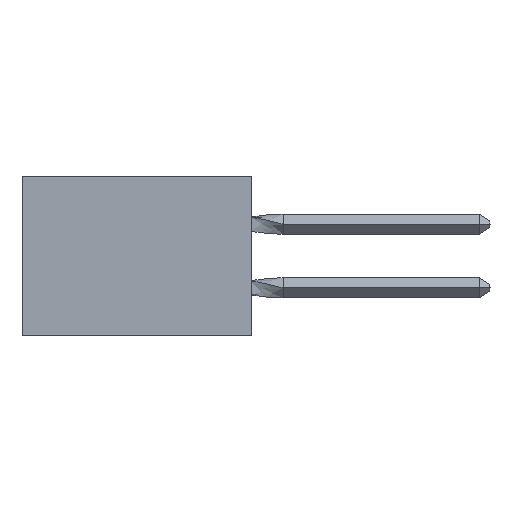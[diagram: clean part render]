
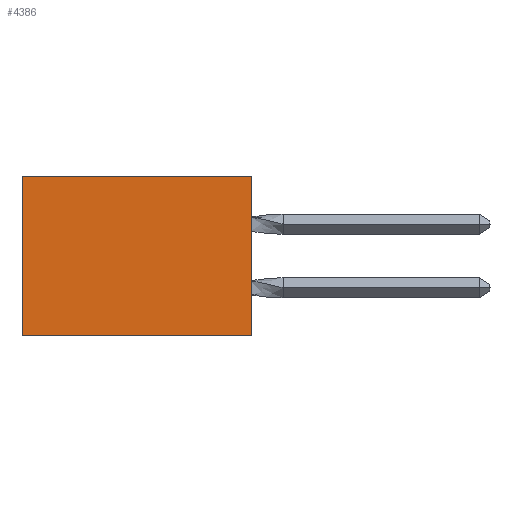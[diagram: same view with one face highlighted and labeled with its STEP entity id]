
A CAD part, left-side view. The second image highlights one B-rep face of the part: STEP entity #4386.
In plain terms, the highlighted planar face has unit normal (-1, 0, 0).
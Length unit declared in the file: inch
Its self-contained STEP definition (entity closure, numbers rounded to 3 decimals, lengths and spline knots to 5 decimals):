
#425 = ORIENTED_EDGE ( 'NONE', *, *, #20568, .T. ) ;
#957 = VERTEX_POINT ( 'NONE', #29753 ) ;
#1136 = LINE ( 'NONE', #21128, #17414 ) ;
#1670 = EDGE_CURVE ( 'NONE', #957, #11367, #22996, .T. ) ;
#1974 = DIRECTION ( 'NONE',  ( 1., 0., 0. ) ) ;
#3544 = DIRECTION ( 'NONE',  ( 0., 0., -1. ) ) ;
#3675 = ORIENTED_EDGE ( 'NONE', *, *, #31284, .F. ) ;
#4386 = ADVANCED_FACE ( 'NONE', ( #19103 ), #10804, .F. ) ;
#4981 = VERTEX_POINT ( 'NONE', #10867 ) ;
#6516 = VECTOR ( 'NONE', #23157, 39.37008 ) ;
#7247 = CARTESIAN_POINT ( 'NONE',  ( 0.305, 0., 0. ) ) ;
#10804 = PLANE ( 'NONE',  #24406 ) ;
#10867 = CARTESIAN_POINT ( 'NONE',  ( 0.305, 0.72, 0. ) ) ;
#11367 = VERTEX_POINT ( 'NONE', #18844 ) ;
#11727 = CARTESIAN_POINT ( 'NONE',  ( 0.305, 0., -0.5 ) ) ;
#15640 = EDGE_CURVE ( 'NONE', #15879, #4981, #16279, .T. ) ;
#15879 = VERTEX_POINT ( 'NONE', #7247 ) ;
#16279 = LINE ( 'NONE', #20066, #6516 ) ;
#16766 = ORIENTED_EDGE ( 'NONE', *, *, #15640, .T. ) ;
#16795 = DIRECTION ( 'NONE',  ( 0., 0., -1. ) ) ;
#17414 = VECTOR ( 'NONE', #3544, 39.37008 ) ;
#18844 = CARTESIAN_POINT ( 'NONE',  ( 0.305, 0.72, -0.5 ) ) ;
#19103 = FACE_OUTER_BOUND ( 'NONE', #37773, .T. ) ;
#20066 = CARTESIAN_POINT ( 'NONE',  ( 0.305, 0., 0. ) ) ;
#20568 = EDGE_CURVE ( 'NONE', #4981, #11367, #33441, .T. ) ;
#20649 = DIRECTION ( 'NONE',  ( 0., 1., 0. ) ) ;
#21128 = CARTESIAN_POINT ( 'NONE',  ( 0.305, 0., -0.5 ) ) ;
#22996 = LINE ( 'NONE', #11727, #23452 ) ;
#23157 = DIRECTION ( 'NONE',  ( 0., 1., 0. ) ) ;
#23452 = VECTOR ( 'NONE', #20649, 39.37008 ) ;
#24406 = AXIS2_PLACEMENT_3D ( 'NONE', #31503, #1974, #16795 ) ;
#26112 = ORIENTED_EDGE ( 'NONE', *, *, #1670, .F. ) ;
#26463 = VECTOR ( 'NONE', #28779, 39.37008 ) ;
#28374 = CARTESIAN_POINT ( 'NONE',  ( 0.305, 0.72, -0.5 ) ) ;
#28779 = DIRECTION ( 'NONE',  ( 0., 0., -1. ) ) ;
#29753 = CARTESIAN_POINT ( 'NONE',  ( 0.305, 0., -0.5 ) ) ;
#31284 = EDGE_CURVE ( 'NONE', #15879, #957, #1136, .T. ) ;
#31503 = CARTESIAN_POINT ( 'NONE',  ( 0.305, 0., -0.5 ) ) ;
#33441 = LINE ( 'NONE', #28374, #26463 ) ;
#37773 = EDGE_LOOP ( 'NONE', ( #425, #26112, #3675, #16766 ) ) ;
